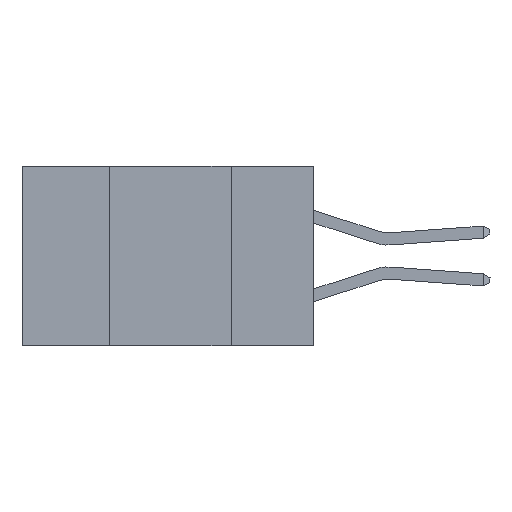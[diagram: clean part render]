
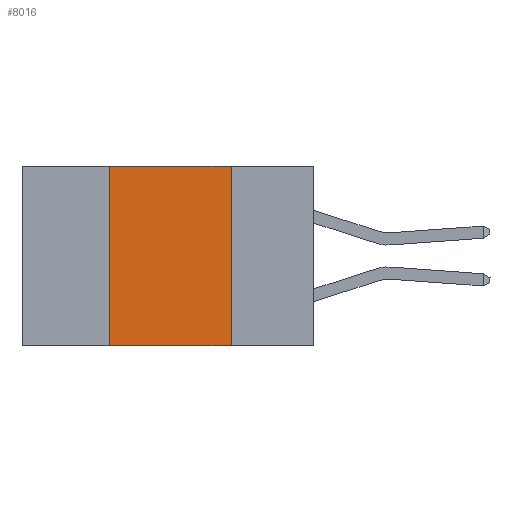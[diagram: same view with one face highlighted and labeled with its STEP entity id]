
A CAD part, left-side view. The second image highlights one B-rep face of the part: STEP entity #8016.
In plain terms, the highlighted planar face has unit normal (-1, 0, 0).
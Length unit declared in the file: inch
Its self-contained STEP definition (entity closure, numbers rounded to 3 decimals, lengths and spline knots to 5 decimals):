
#511 = ORIENTED_EDGE ( 'NONE', *, *, #14734, .F. ) ;
#598 = VERTEX_POINT ( 'NONE', #2943 ) ;
#1138 = DIRECTION ( 'NONE',  ( 0., -1., 0. ) ) ;
#1873 = EDGE_LOOP ( 'NONE', ( #4935, #5531, #511, #9265 ) ) ;
#1939 = CARTESIAN_POINT ( 'NONE',  ( 0., 0.17, 0. ) ) ;
#2023 = CARTESIAN_POINT ( 'NONE',  ( 0., 0.42, 0. ) ) ;
#2257 = PLANE ( 'NONE',  #17280 ) ;
#2585 = VECTOR ( 'NONE', #1138, 39.37008 ) ;
#2943 = CARTESIAN_POINT ( 'NONE',  ( 0., 0.42, 0. ) ) ;
#3310 = FACE_OUTER_BOUND ( 'NONE', #1873, .T. ) ;
#3540 = CARTESIAN_POINT ( 'NONE',  ( 0., 0.17, 0. ) ) ;
#3602 = DIRECTION ( 'NONE',  ( 1., 0., 0. ) ) ;
#3856 = VERTEX_POINT ( 'NONE', #7356 ) ;
#3999 = VECTOR ( 'NONE', #12882, 39.37008 ) ;
#4935 = ORIENTED_EDGE ( 'NONE', *, *, #12922, .F. ) ;
#5134 = VERTEX_POINT ( 'NONE', #1939 ) ;
#5235 = DIRECTION ( 'NONE',  ( 0., -1., 0. ) ) ;
#5397 = EDGE_CURVE ( 'NONE', #16828, #3856, #9600, .T. ) ;
#5531 = ORIENTED_EDGE ( 'NONE', *, *, #10073, .F. ) ;
#7049 = LINE ( 'NONE', #3540, #3999 ) ;
#7356 = CARTESIAN_POINT ( 'NONE',  ( 0., 0.17, -0.37 ) ) ;
#8016 = ADVANCED_FACE ( 'NONE', ( #3310 ), #2257, .F. ) ;
#8695 = VECTOR ( 'NONE', #15442, 39.37008 ) ;
#9265 = ORIENTED_EDGE ( 'NONE', *, *, #5397, .T. ) ;
#9600 = LINE ( 'NONE', #11859, #2585 ) ;
#10073 = EDGE_CURVE ( 'NONE', #598, #5134, #17127, .T. ) ;
#10477 = CARTESIAN_POINT ( 'NONE',  ( 0., 0.6, 0. ) ) ;
#11576 = CARTESIAN_POINT ( 'NONE',  ( 0., 0.6, 0. ) ) ;
#11859 = CARTESIAN_POINT ( 'NONE',  ( 0., 0.6, -0.37 ) ) ;
#12728 = LINE ( 'NONE', #2023, #8695 ) ;
#12882 = DIRECTION ( 'NONE',  ( 0., 0., -1. ) ) ;
#12922 = EDGE_CURVE ( 'NONE', #5134, #3856, #7049, .T. ) ;
#12951 = DIRECTION ( 'NONE',  ( 0., 0., -1. ) ) ;
#13999 = CARTESIAN_POINT ( 'NONE',  ( 0., 0.42, -0.37 ) ) ;
#14734 = EDGE_CURVE ( 'NONE', #16828, #598, #12728, .T. ) ;
#15442 = DIRECTION ( 'NONE',  ( 0., 0., 1. ) ) ;
#15848 = VECTOR ( 'NONE', #5235, 39.37008 ) ;
#16828 = VERTEX_POINT ( 'NONE', #13999 ) ;
#17127 = LINE ( 'NONE', #10477, #15848 ) ;
#17280 = AXIS2_PLACEMENT_3D ( 'NONE', #11576, #3602, #12951 ) ;
